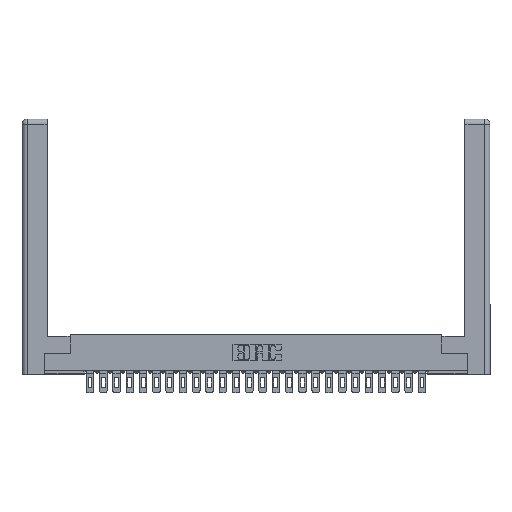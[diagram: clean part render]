
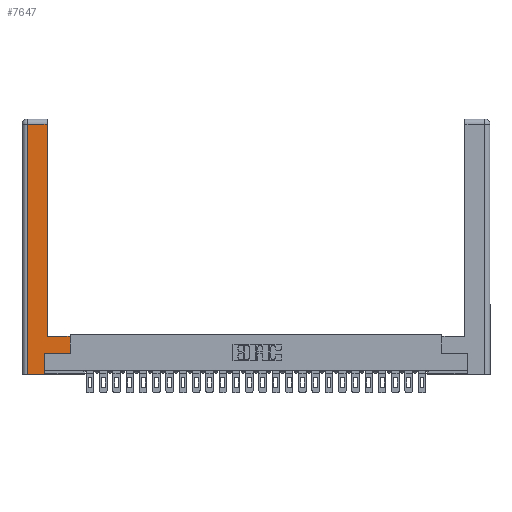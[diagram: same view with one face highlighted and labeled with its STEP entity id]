
A CAD part, top view. The second image highlights one B-rep face of the part: STEP entity #7647.
In plain terms, the highlighted planar face has unit normal (0, 0, 1).
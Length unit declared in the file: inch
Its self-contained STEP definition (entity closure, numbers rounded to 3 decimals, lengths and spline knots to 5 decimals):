
#134 = VERTEX_POINT ( 'NONE', #3616 ) ;
#150 = VECTOR ( 'NONE', #4702, 39.37008 ) ;
#468 = DIRECTION ( 'NONE',  ( -1., 0., 0. ) ) ;
#783 = AXIS2_PLACEMENT_3D ( 'NONE', #20174, #1063, #24281 ) ;
#915 = CARTESIAN_POINT ( 'NONE',  ( 0.0615, 0., 0. ) ) ;
#1063 = DIRECTION ( 'NONE',  ( 0., 0., -1. ) ) ;
#1237 = CARTESIAN_POINT ( 'NONE',  ( 0.265, 0., 0. ) ) ;
#1883 = EDGE_CURVE ( 'NONE', #134, #24498, #11874, .T. ) ;
#2753 = VERTEX_POINT ( 'NONE', #19749 ) ;
#3333 = LINE ( 'NONE', #19341, #20690 ) ;
#3573 = CARTESIAN_POINT ( 'NONE',  ( 0.265, 0.245, 0. ) ) ;
#3616 = CARTESIAN_POINT ( 'NONE',  ( 0.0615, 2.94, 0. ) ) ;
#4169 = ORIENTED_EDGE ( 'NONE', *, *, #1883, .T. ) ;
#4702 = DIRECTION ( 'NONE',  ( 0., -1., 0. ) ) ;
#5033 = CARTESIAN_POINT ( 'NONE',  ( 0.0615, 2.94, 0. ) ) ;
#5069 = CARTESIAN_POINT ( 'NONE',  ( 0.0615, 0., 0. ) ) ;
#6148 = VECTOR ( 'NONE', #23534, 39.37008 ) ;
#6800 = LINE ( 'NONE', #17760, #14127 ) ;
#7647 = ADVANCED_FACE ( 'NONE', ( #18316 ), #24569, .F. ) ;
#8489 = ORIENTED_EDGE ( 'NONE', *, *, #19533, .T. ) ;
#8871 = LINE ( 'NONE', #5033, #26153 ) ;
#9297 = CARTESIAN_POINT ( 'NONE',  ( 0.295, 2.94, 0. ) ) ;
#9726 = EDGE_CURVE ( 'NONE', #24618, #2753, #22466, .T. ) ;
#10053 = EDGE_CURVE ( 'NONE', #24498, #16566, #17731, .T. ) ;
#10065 = EDGE_CURVE ( 'NONE', #2753, #10682, #25772, .T. ) ;
#10480 = VERTEX_POINT ( 'NONE', #12664 ) ;
#10628 = VERTEX_POINT ( 'NONE', #16279 ) ;
#10682 = VERTEX_POINT ( 'NONE', #9297 ) ;
#10705 = ORIENTED_EDGE ( 'NONE', *, *, #19390, .T. ) ;
#11874 = LINE ( 'NONE', #5069, #150 ) ;
#12124 = ORIENTED_EDGE ( 'NONE', *, *, #23043, .T. ) ;
#12664 = CARTESIAN_POINT ( 'NONE',  ( 0.565, 0.245, 0. ) ) ;
#12745 = ORIENTED_EDGE ( 'NONE', *, *, #10065, .T. ) ;
#12802 = LINE ( 'NONE', #3573, #23776 ) ;
#13070 = CARTESIAN_POINT ( 'NONE',  ( 0.295, 3., 0. ) ) ;
#14127 = VECTOR ( 'NONE', #16017, 39.37008 ) ;
#16017 = DIRECTION ( 'NONE',  ( 0., 1., 0. ) ) ;
#16191 = ORIENTED_EDGE ( 'NONE', *, *, #9726, .T. ) ;
#16244 = EDGE_LOOP ( 'NONE', ( #12745, #12124, #4169, #26398, #8489, #19636, #10705, #16191 ) ) ;
#16279 = CARTESIAN_POINT ( 'NONE',  ( 0.265, 0.245, 0. ) ) ;
#16566 = VERTEX_POINT ( 'NONE', #1237 ) ;
#17350 = DIRECTION ( 'NONE',  ( 0., 1., 0. ) ) ;
#17424 = VECTOR ( 'NONE', #468, 39.37008 ) ;
#17731 = LINE ( 'NONE', #21313, #6148 ) ;
#17760 = CARTESIAN_POINT ( 'NONE',  ( 0.565, 0.45, 0. ) ) ;
#18316 = FACE_OUTER_BOUND ( 'NONE', #16244, .T. ) ;
#19341 = CARTESIAN_POINT ( 'NONE',  ( 0.565, 0.245, 0. ) ) ;
#19390 = EDGE_CURVE ( 'NONE', #10480, #24618, #6800, .T. ) ;
#19533 = EDGE_CURVE ( 'NONE', #16566, #10628, #12802, .T. ) ;
#19636 = ORIENTED_EDGE ( 'NONE', *, *, #21619, .T. ) ;
#19749 = CARTESIAN_POINT ( 'NONE',  ( 0.295, 0.45, 0. ) ) ;
#20174 = CARTESIAN_POINT ( 'NONE',  ( 0., 0., 0. ) ) ;
#20690 = VECTOR ( 'NONE', #25527, 39.37008 ) ;
#21313 = CARTESIAN_POINT ( 'NONE',  ( 0.265, 0., 0. ) ) ;
#21619 = EDGE_CURVE ( 'NONE', #10628, #10480, #3333, .T. ) ;
#22466 = LINE ( 'NONE', #26054, #17424 ) ;
#23043 = EDGE_CURVE ( 'NONE', #10682, #134, #8871, .T. ) ;
#23131 = VECTOR ( 'NONE', #17350, 39.37008 ) ;
#23534 = DIRECTION ( 'NONE',  ( 1., 0., 0. ) ) ;
#23776 = VECTOR ( 'NONE', #25178, 39.37008 ) ;
#24281 = DIRECTION ( 'NONE',  ( -1., 0., 0. ) ) ;
#24498 = VERTEX_POINT ( 'NONE', #915 ) ;
#24569 = PLANE ( 'NONE',  #783 ) ;
#24594 = DIRECTION ( 'NONE',  ( -1., 0., 0. ) ) ;
#24618 = VERTEX_POINT ( 'NONE', #25006 ) ;
#25006 = CARTESIAN_POINT ( 'NONE',  ( 0.565, 0.45, 0. ) ) ;
#25178 = DIRECTION ( 'NONE',  ( 0., 1., 0. ) ) ;
#25527 = DIRECTION ( 'NONE',  ( 1., 0., 0. ) ) ;
#25772 = LINE ( 'NONE', #13070, #23131 ) ;
#26054 = CARTESIAN_POINT ( 'NONE',  ( 0.295, 0.45, 0. ) ) ;
#26153 = VECTOR ( 'NONE', #24594, 39.37008 ) ;
#26398 = ORIENTED_EDGE ( 'NONE', *, *, #10053, .T. ) ;
